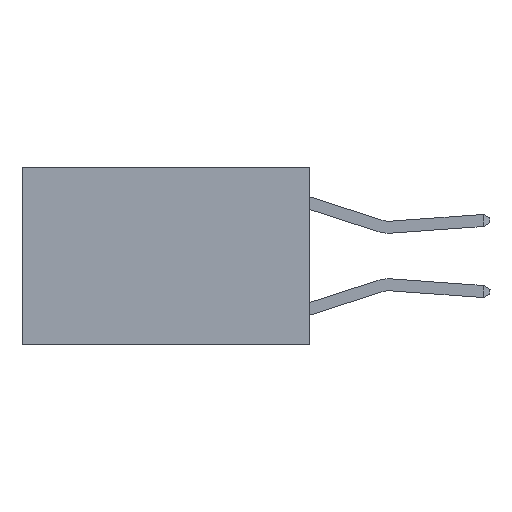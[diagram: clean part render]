
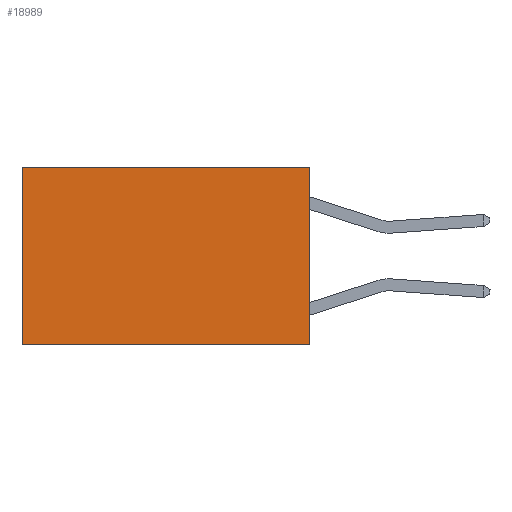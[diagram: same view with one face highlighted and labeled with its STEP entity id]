
A CAD part, left-side view. The second image highlights one B-rep face of the part: STEP entity #18989.
In plain terms, the highlighted planar face has unit normal (-1, 0, 0).
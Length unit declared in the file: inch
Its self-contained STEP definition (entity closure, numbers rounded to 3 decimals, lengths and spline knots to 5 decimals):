
#46 = ORIENTED_EDGE ( 'NONE', *, *, #22794, .F. ) ;
#1421 = LINE ( 'NONE', #1897, #22438 ) ;
#1890 = CARTESIAN_POINT ( 'NONE',  ( 0.2625, 0., 0. ) ) ;
#1897 = CARTESIAN_POINT ( 'NONE',  ( 0.2625, 0.6, 0. ) ) ;
#3988 = VECTOR ( 'NONE', #7154, 39.37008 ) ;
#4027 = DIRECTION ( 'NONE',  ( 0., 0., -1. ) ) ;
#4545 = LINE ( 'NONE', #23397, #8711 ) ;
#5280 = VERTEX_POINT ( 'NONE', #14748 ) ;
#6083 = VECTOR ( 'NONE', #19149, 39.37008 ) ;
#6709 = ORIENTED_EDGE ( 'NONE', *, *, #25670, .F. ) ;
#7040 = EDGE_CURVE ( 'NONE', #7501, #10883, #1421, .T. ) ;
#7154 = DIRECTION ( 'NONE',  ( 0., 0., -1. ) ) ;
#7382 = CARTESIAN_POINT ( 'NONE',  ( 0.2625, 0., 0. ) ) ;
#7501 = VERTEX_POINT ( 'NONE', #18037 ) ;
#8711 = VECTOR ( 'NONE', #11397, 39.37008 ) ;
#9184 = EDGE_LOOP ( 'NONE', ( #13636, #46, #6709, #24605 ) ) ;
#9433 = DIRECTION ( 'NONE',  ( 0., 0., -1. ) ) ;
#10883 = VERTEX_POINT ( 'NONE', #18160 ) ;
#11397 = DIRECTION ( 'NONE',  ( 0., 1., 0. ) ) ;
#13216 = CARTESIAN_POINT ( 'NONE',  ( 0.2625, 0., 0. ) ) ;
#13636 = ORIENTED_EDGE ( 'NONE', *, *, #7040, .T. ) ;
#14599 = EDGE_CURVE ( 'NONE', #19232, #7501, #4545, .T. ) ;
#14748 = CARTESIAN_POINT ( 'NONE',  ( 0.2625, 0., -0.37 ) ) ;
#18037 = CARTESIAN_POINT ( 'NONE',  ( 0.2625, 0.6, 0. ) ) ;
#18160 = CARTESIAN_POINT ( 'NONE',  ( 0.2625, 0.6, -0.37 ) ) ;
#18720 = FACE_OUTER_BOUND ( 'NONE', #9184, .T. ) ;
#18989 = ADVANCED_FACE ( 'NONE', ( #18720 ), #25379, .F. ) ;
#19149 = DIRECTION ( 'NONE',  ( 0., 1., 0. ) ) ;
#19232 = VERTEX_POINT ( 'NONE', #1890 ) ;
#21485 = DIRECTION ( 'NONE',  ( 1., 0., 0. ) ) ;
#22200 = LINE ( 'NONE', #25059, #6083 ) ;
#22438 = VECTOR ( 'NONE', #4027, 39.37008 ) ;
#22613 = AXIS2_PLACEMENT_3D ( 'NONE', #7382, #21485, #9433 ) ;
#22794 = EDGE_CURVE ( 'NONE', #5280, #10883, #22200, .T. ) ;
#23397 = CARTESIAN_POINT ( 'NONE',  ( 0.2625, 0., 0. ) ) ;
#24605 = ORIENTED_EDGE ( 'NONE', *, *, #14599, .T. ) ;
#25059 = CARTESIAN_POINT ( 'NONE',  ( 0.2625, 0., -0.37 ) ) ;
#25379 = PLANE ( 'NONE',  #22613 ) ;
#25442 = LINE ( 'NONE', #13216, #3988 ) ;
#25670 = EDGE_CURVE ( 'NONE', #19232, #5280, #25442, .T. ) ;
